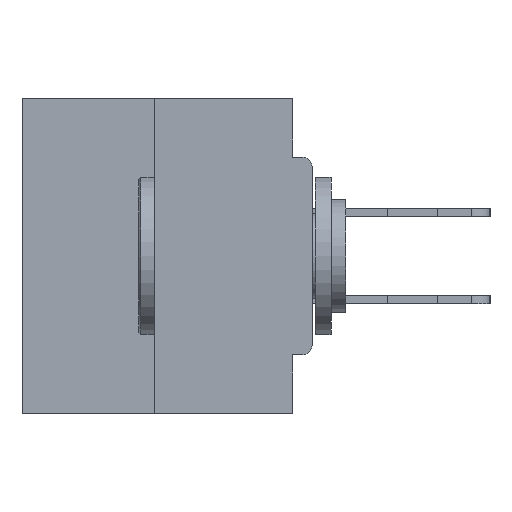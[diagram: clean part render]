
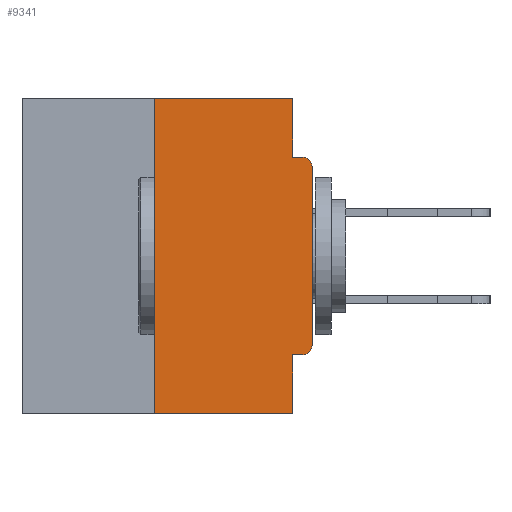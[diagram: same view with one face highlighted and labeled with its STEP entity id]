
A CAD part, left-side view. The second image highlights one B-rep face of the part: STEP entity #9341.
In plain terms, the highlighted planar face has unit normal (-1, 0, 0).
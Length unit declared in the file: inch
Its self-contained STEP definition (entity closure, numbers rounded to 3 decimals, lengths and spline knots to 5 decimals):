
#227 = LINE ( 'NONE', #11232, #33629 ) ;
#764 = LINE ( 'NONE', #3246, #26823 ) ;
#1321 = ORIENTED_EDGE ( 'NONE', *, *, #3800, .F. ) ;
#2109 = VERTEX_POINT ( 'NONE', #34819 ) ;
#3152 = CARTESIAN_POINT ( 'NONE',  ( 0., 0.46, 0. ) ) ;
#3246 = CARTESIAN_POINT ( 'NONE',  ( 0., 0.46, -0.5 ) ) ;
#3634 = LINE ( 'NONE', #36352, #33857 ) ;
#3800 = EDGE_CURVE ( 'NONE', #31607, #31443, #3634, .T. ) ;
#4025 = DIRECTION ( 'NONE',  ( 0., 0., -1. ) ) ;
#4209 = DIRECTION ( 'NONE',  ( 0., 0., -1. ) ) ;
#4222 = VERTEX_POINT ( 'NONE', #12692 ) ;
#4379 = CARTESIAN_POINT ( 'NONE',  ( 0., 0., -0.3915 ) ) ;
#4405 = ORIENTED_EDGE ( 'NONE', *, *, #14903, .T. ) ;
#6402 = CARTESIAN_POINT ( 'NONE',  ( 0., 0.031, -0.0935 ) ) ;
#7266 = DIRECTION ( 'NONE',  ( 1., 0., 0. ) ) ;
#7811 = VECTOR ( 'NONE', #10338, 39.37008 ) ;
#8560 = LINE ( 'NONE', #29310, #22266 ) ;
#9192 = VERTEX_POINT ( 'NONE', #6402 ) ;
#9311 = VERTEX_POINT ( 'NONE', #30581 ) ;
#9334 = AXIS2_PLACEMENT_3D ( 'NONE', #18544, #7266, #4209 ) ;
#9341 = ADVANCED_FACE ( 'NONE', ( #27727 ), #21477, .F. ) ;
#9518 = DIRECTION ( 'NONE',  ( 0., -1., 0. ) ) ;
#9819 = EDGE_CURVE ( 'NONE', #2109, #9192, #30028, .T. ) ;
#10161 = EDGE_LOOP ( 'NONE', ( #17406, #26888, #22195, #26816, #1321, #4405, #26865, #26889, #29206, #16452 ) ) ;
#10338 = DIRECTION ( 'NONE',  ( 0., 0., 1. ) ) ;
#10549 = EDGE_CURVE ( 'NONE', #31443, #11945, #227, .T. ) ;
#11232 = CARTESIAN_POINT ( 'NONE',  ( 0., 0.031, -0.5 ) ) ;
#11945 = VERTEX_POINT ( 'NONE', #21072 ) ;
#12692 = CARTESIAN_POINT ( 'NONE',  ( 0., 0.25, 0. ) ) ;
#13030 = VECTOR ( 'NONE', #4025, 39.37008 ) ;
#13471 = VERTEX_POINT ( 'NONE', #4379 ) ;
#14842 = CARTESIAN_POINT ( 'NONE',  ( 0., 0.015, -0.3915 ) ) ;
#14903 = EDGE_CURVE ( 'NONE', #31607, #13471, #27417, .T. ) ;
#15213 = DIRECTION ( 'NONE',  ( 0., -1., 0. ) ) ;
#16452 = ORIENTED_EDGE ( 'NONE', *, *, #9819, .F. ) ;
#16954 = CARTESIAN_POINT ( 'NONE',  ( 0., 0., 0. ) ) ;
#17406 = ORIENTED_EDGE ( 'NONE', *, *, #22796, .F. ) ;
#17795 = DIRECTION ( 'NONE',  ( 0., 0., -1. ) ) ;
#18048 = CARTESIAN_POINT ( 'NONE',  ( 0., 0.015, -0.1085 ) ) ;
#18207 = EDGE_CURVE ( 'NONE', #9311, #33394, #37693, .T. ) ;
#18544 = CARTESIAN_POINT ( 'NONE',  ( 0., 0.46, 0. ) ) ;
#20071 = CARTESIAN_POINT ( 'NONE',  ( 0., 0.015, -0.4065 ) ) ;
#21000 = DIRECTION ( 'NONE',  ( -1., 0., 0. ) ) ;
#21072 = CARTESIAN_POINT ( 'NONE',  ( 0., 0.031, -0.5 ) ) ;
#21477 = PLANE ( 'NONE',  #9334 ) ;
#21721 = VERTEX_POINT ( 'NONE', #33775 ) ;
#22195 = ORIENTED_EDGE ( 'NONE', *, *, #35056, .T. ) ;
#22266 = VECTOR ( 'NONE', #35360, 39.37008 ) ;
#22796 = EDGE_CURVE ( 'NONE', #4222, #2109, #35363, .T. ) ;
#24315 = CARTESIAN_POINT ( 'NONE',  ( 0., 0.015, -0.0935 ) ) ;
#25422 = CARTESIAN_POINT ( 'NONE',  ( 0., 0.25, 0. ) ) ;
#25653 = LINE ( 'NONE', #25422, #7811 ) ;
#25786 = AXIS2_PLACEMENT_3D ( 'NONE', #14842, #35391, #17795 ) ;
#25865 = VECTOR ( 'NONE', #37484, 39.37008 ) ;
#26816 = ORIENTED_EDGE ( 'NONE', *, *, #10549, .F. ) ;
#26823 = VECTOR ( 'NONE', #15213, 39.37008 ) ;
#26865 = ORIENTED_EDGE ( 'NONE', *, *, #31940, .T. ) ;
#26888 = ORIENTED_EDGE ( 'NONE', *, *, #27885, .F. ) ;
#26889 = ORIENTED_EDGE ( 'NONE', *, *, #18207, .T. ) ;
#27417 = CIRCLE ( 'NONE', #25786, 0.015 ) ;
#27727 = FACE_OUTER_BOUND ( 'NONE', #10161, .T. ) ;
#27885 = EDGE_CURVE ( 'NONE', #21721, #4222, #25653, .T. ) ;
#29206 = ORIENTED_EDGE ( 'NONE', *, *, #30015, .F. ) ;
#29310 = CARTESIAN_POINT ( 'NONE',  ( 0., 0., -0.0935 ) ) ;
#29984 = DIRECTION ( 'NONE',  ( 0., 0., -1. ) ) ;
#30008 = LINE ( 'NONE', #16954, #25865 ) ;
#30015 = EDGE_CURVE ( 'NONE', #9192, #33394, #8560, .T. ) ;
#30028 = LINE ( 'NONE', #36051, #13030 ) ;
#30581 = CARTESIAN_POINT ( 'NONE',  ( 0., 0., -0.1085 ) ) ;
#31443 = VERTEX_POINT ( 'NONE', #33937 ) ;
#31607 = VERTEX_POINT ( 'NONE', #20071 ) ;
#31940 = EDGE_CURVE ( 'NONE', #13471, #9311, #30008, .T. ) ;
#33006 = AXIS2_PLACEMENT_3D ( 'NONE', #18048, #21000, #29984 ) ;
#33394 = VERTEX_POINT ( 'NONE', #24315 ) ;
#33398 = DIRECTION ( 'NONE',  ( 0., 1., 0. ) ) ;
#33525 = VECTOR ( 'NONE', #9518, 39.37008 ) ;
#33629 = VECTOR ( 'NONE', #37631, 39.37008 ) ;
#33775 = CARTESIAN_POINT ( 'NONE',  ( 0., 0.25, -0.5 ) ) ;
#33857 = VECTOR ( 'NONE', #33398, 39.37008 ) ;
#33937 = CARTESIAN_POINT ( 'NONE',  ( 0., 0.031, -0.4065 ) ) ;
#34819 = CARTESIAN_POINT ( 'NONE',  ( 0., 0.031, 0. ) ) ;
#35056 = EDGE_CURVE ( 'NONE', #21721, #11945, #764, .T. ) ;
#35360 = DIRECTION ( 'NONE',  ( 0., -1., 0. ) ) ;
#35363 = LINE ( 'NONE', #3152, #33525 ) ;
#35391 = DIRECTION ( 'NONE',  ( -1., 0., 0. ) ) ;
#36051 = CARTESIAN_POINT ( 'NONE',  ( 0., 0.031, 0. ) ) ;
#36352 = CARTESIAN_POINT ( 'NONE',  ( 0., 0., -0.4065 ) ) ;
#37484 = DIRECTION ( 'NONE',  ( 0., 0., 1. ) ) ;
#37631 = DIRECTION ( 'NONE',  ( 0., 0., -1. ) ) ;
#37693 = CIRCLE ( 'NONE', #33006, 0.015 ) ;
